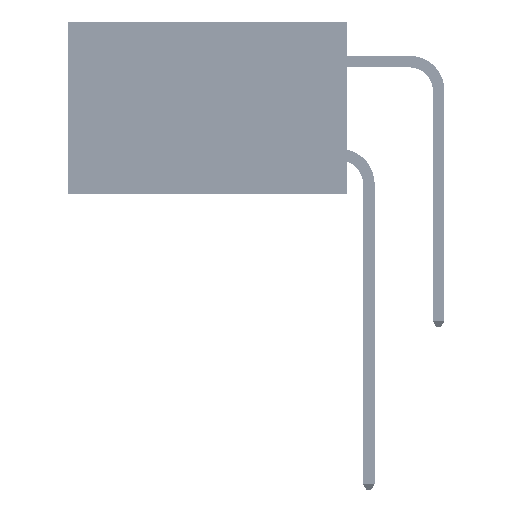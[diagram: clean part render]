
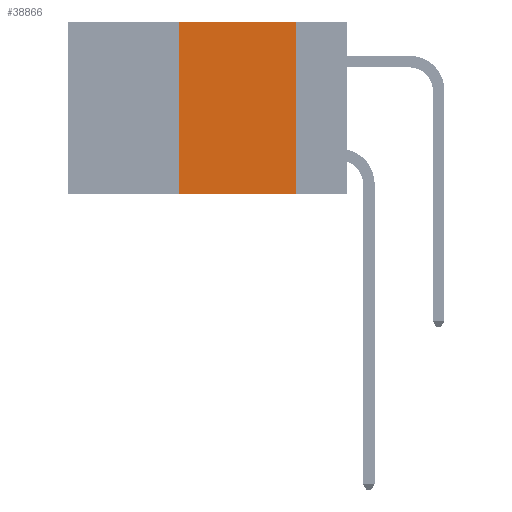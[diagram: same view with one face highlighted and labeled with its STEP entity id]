
A CAD part, left-side view. The second image highlights one B-rep face of the part: STEP entity #38866.
In plain terms, the highlighted planar face has unit normal (-1, 0, 0).
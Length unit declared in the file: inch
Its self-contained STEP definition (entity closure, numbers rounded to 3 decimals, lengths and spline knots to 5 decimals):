
#1079 = EDGE_CURVE ( 'NONE', #35879, #12656, #22167, .T. ) ;
#2732 = ORIENTED_EDGE ( 'NONE', *, *, #40594, .T. ) ;
#3659 = CARTESIAN_POINT ( 'NONE',  ( 0., 0.6, -0.37 ) ) ;
#5451 = EDGE_CURVE ( 'NONE', #12656, #18445, #46933, .T. ) ;
#5814 = LINE ( 'NONE', #9876, #48635 ) ;
#7355 = VECTOR ( 'NONE', #43256, 39.37008 ) ;
#7795 = DIRECTION ( 'NONE',  ( 0., 0., -1. ) ) ;
#8356 = CARTESIAN_POINT ( 'NONE',  ( 0., 0.6, 0. ) ) ;
#9331 = EDGE_CURVE ( 'NONE', #18445, #40975, #5814, .T. ) ;
#9876 = CARTESIAN_POINT ( 'NONE',  ( 0., 0.11, 0. ) ) ;
#10268 = VECTOR ( 'NONE', #47427, 39.37008 ) ;
#10476 = CARTESIAN_POINT ( 'NONE',  ( 0., 0.11, -0.37 ) ) ;
#11142 = ORIENTED_EDGE ( 'NONE', *, *, #1079, .F. ) ;
#12656 = VERTEX_POINT ( 'NONE', #46602 ) ;
#14548 = DIRECTION ( 'NONE',  ( 0., 0., 1. ) ) ;
#17416 = CARTESIAN_POINT ( 'NONE',  ( 0., 0.11, 0. ) ) ;
#17744 = ORIENTED_EDGE ( 'NONE', *, *, #9331, .F. ) ;
#18445 = VERTEX_POINT ( 'NONE', #17416 ) ;
#18682 = LINE ( 'NONE', #3659, #7355 ) ;
#19227 = CARTESIAN_POINT ( 'NONE',  ( 0., 0.6, 0. ) ) ;
#19393 = AXIS2_PLACEMENT_3D ( 'NONE', #19227, #20236, #7795 ) ;
#20236 = DIRECTION ( 'NONE',  ( 1., 0., 0. ) ) ;
#22167 = LINE ( 'NONE', #49283, #40701 ) ;
#26305 = ORIENTED_EDGE ( 'NONE', *, *, #5451, .F. ) ;
#26910 = EDGE_LOOP ( 'NONE', ( #17744, #26305, #11142, #2732 ) ) ;
#28434 = DIRECTION ( 'NONE',  ( 0., 0., -1. ) ) ;
#30240 = CARTESIAN_POINT ( 'NONE',  ( 0., 0.36, -0.37 ) ) ;
#34714 = PLANE ( 'NONE',  #19393 ) ;
#35879 = VERTEX_POINT ( 'NONE', #30240 ) ;
#38866 = ADVANCED_FACE ( 'NONE', ( #43308 ), #34714, .F. ) ;
#40594 = EDGE_CURVE ( 'NONE', #35879, #40975, #18682, .T. ) ;
#40701 = VECTOR ( 'NONE', #14548, 39.37008 ) ;
#40975 = VERTEX_POINT ( 'NONE', #10476 ) ;
#43256 = DIRECTION ( 'NONE',  ( 0., -1., 0. ) ) ;
#43308 = FACE_OUTER_BOUND ( 'NONE', #26910, .T. ) ;
#46602 = CARTESIAN_POINT ( 'NONE',  ( 0., 0.36, 0. ) ) ;
#46933 = LINE ( 'NONE', #8356, #10268 ) ;
#47427 = DIRECTION ( 'NONE',  ( 0., -1., 0. ) ) ;
#48635 = VECTOR ( 'NONE', #28434, 39.37008 ) ;
#49283 = CARTESIAN_POINT ( 'NONE',  ( 0., 0.36, 0. ) ) ;
